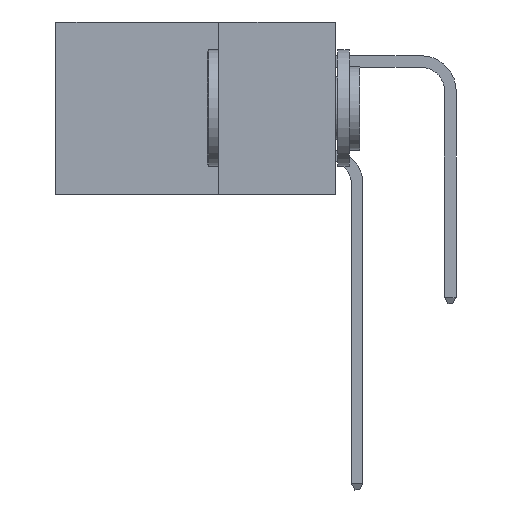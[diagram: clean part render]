
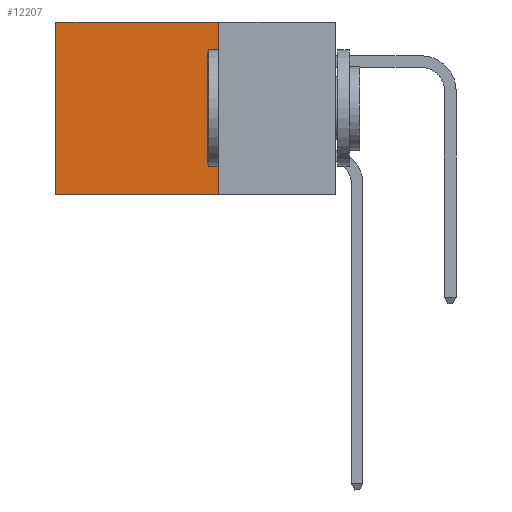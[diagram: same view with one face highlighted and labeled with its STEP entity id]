
A CAD part, left-side view. The second image highlights one B-rep face of the part: STEP entity #12207.
In plain terms, the highlighted planar face has unit normal (-1, 0, 0).
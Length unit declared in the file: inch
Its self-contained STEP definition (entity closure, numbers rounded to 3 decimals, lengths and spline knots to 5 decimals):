
#104 = AXIS2_PLACEMENT_3D ( 'NONE', #7975, #5493, #14170 ) ;
#630 = LINE ( 'NONE', #2022, #13837 ) ;
#2022 = CARTESIAN_POINT ( 'NONE',  ( 0.2875, 0.6, 0. ) ) ;
#2120 = VECTOR ( 'NONE', #14948, 39.37008 ) ;
#2224 = CARTESIAN_POINT ( 'NONE',  ( 0.2875, 0.25, 0. ) ) ;
#3000 = VECTOR ( 'NONE', #3587, 39.37008 ) ;
#3456 = DIRECTION ( 'NONE',  ( 0., 1., 0. ) ) ;
#3587 = DIRECTION ( 'NONE',  ( 0., 1., 0. ) ) ;
#3687 = CARTESIAN_POINT ( 'NONE',  ( 0.2875, 0.25, 0. ) ) ;
#5493 = DIRECTION ( 'NONE',  ( 1., 0., 0. ) ) ;
#7018 = VERTEX_POINT ( 'NONE', #12889 ) ;
#7625 = ORIENTED_EDGE ( 'NONE', *, *, #10024, .T. ) ;
#7760 = VERTEX_POINT ( 'NONE', #14214 ) ;
#7975 = CARTESIAN_POINT ( 'NONE',  ( 0.2875, 0.25, 0. ) ) ;
#8173 = ORIENTED_EDGE ( 'NONE', *, *, #12585, .F. ) ;
#8590 = DIRECTION ( 'NONE',  ( 0., 0., -1. ) ) ;
#9027 = ORIENTED_EDGE ( 'NONE', *, *, #10627, .F. ) ;
#9048 = LINE ( 'NONE', #3687, #2120 ) ;
#9127 = ORIENTED_EDGE ( 'NONE', *, *, #12454, .T. ) ;
#10024 = EDGE_CURVE ( 'NONE', #7760, #15245, #13121, .T. ) ;
#10627 = EDGE_CURVE ( 'NONE', #13753, #7018, #10775, .T. ) ;
#10775 = LINE ( 'NONE', #13539, #13654 ) ;
#12207 = ADVANCED_FACE ( 'NONE', ( #14413 ), #12975, .F. ) ;
#12443 = CARTESIAN_POINT ( 'NONE',  ( 0.2875, 0.6, 0. ) ) ;
#12454 = EDGE_CURVE ( 'NONE', #15245, #7018, #630, .T. ) ;
#12467 = EDGE_LOOP ( 'NONE', ( #9127, #9027, #8173, #7625 ) ) ;
#12585 = EDGE_CURVE ( 'NONE', #7760, #13753, #9048, .T. ) ;
#12889 = CARTESIAN_POINT ( 'NONE',  ( 0.2875, 0.6, -0.37 ) ) ;
#12975 = PLANE ( 'NONE',  #104 ) ;
#13121 = LINE ( 'NONE', #2224, #3000 ) ;
#13539 = CARTESIAN_POINT ( 'NONE',  ( 0.2875, 0.25, -0.37 ) ) ;
#13654 = VECTOR ( 'NONE', #3456, 39.37008 ) ;
#13753 = VERTEX_POINT ( 'NONE', #15991 ) ;
#13837 = VECTOR ( 'NONE', #8590, 39.37008 ) ;
#14170 = DIRECTION ( 'NONE',  ( 0., 0., -1. ) ) ;
#14214 = CARTESIAN_POINT ( 'NONE',  ( 0.2875, 0.25, 0. ) ) ;
#14413 = FACE_OUTER_BOUND ( 'NONE', #12467, .T. ) ;
#14948 = DIRECTION ( 'NONE',  ( 0., 0., -1. ) ) ;
#15245 = VERTEX_POINT ( 'NONE', #12443 ) ;
#15991 = CARTESIAN_POINT ( 'NONE',  ( 0.2875, 0.25, -0.37 ) ) ;
